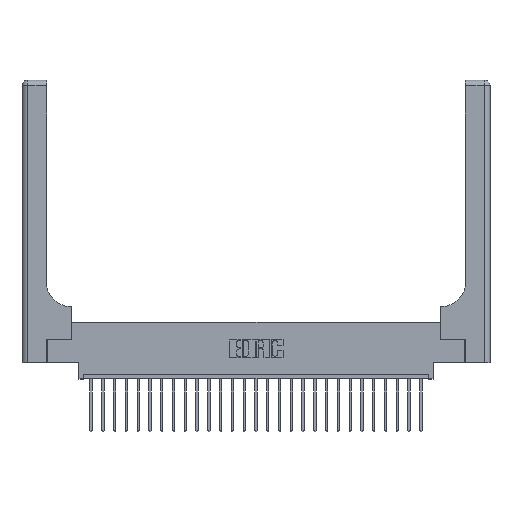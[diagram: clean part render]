
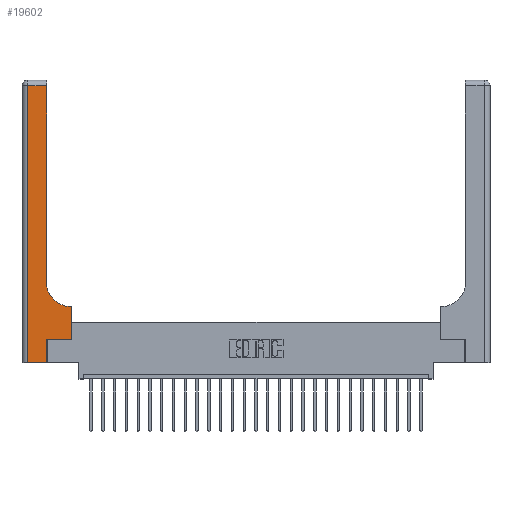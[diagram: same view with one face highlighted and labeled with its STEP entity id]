
A CAD part, top view. The second image highlights one B-rep face of the part: STEP entity #19602.
In plain terms, the highlighted planar face has unit normal (0, 0, 1).
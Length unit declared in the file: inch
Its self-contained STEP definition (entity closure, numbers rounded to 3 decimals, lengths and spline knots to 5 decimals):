
#7 = VERTEX_POINT ( 'NONE', #24614 ) ;
#90 = LINE ( 'NONE', #17116, #2806 ) ;
#502 = VERTEX_POINT ( 'NONE', #16715 ) ;
#616 = PLANE ( 'NONE',  #24711 ) ;
#1683 = ORIENTED_EDGE ( 'NONE', *, *, #7951, .T. ) ;
#2126 = DIRECTION ( 'NONE',  ( 0., 1., 0. ) ) ;
#2358 = LINE ( 'NONE', #4135, #21778 ) ;
#2382 = CARTESIAN_POINT ( 'NONE',  ( 0., 3., 0.37 ) ) ;
#2388 = CARTESIAN_POINT ( 'NONE',  ( 0.528, 0.6, 0.37 ) ) ;
#2448 = CARTESIAN_POINT ( 'NONE',  ( 0.06, 0., 0.37 ) ) ;
#2623 = VECTOR ( 'NONE', #8365, 39.37008 ) ;
#2806 = VECTOR ( 'NONE', #23142, 39.37008 ) ;
#3289 = VECTOR ( 'NONE', #11785, 39.37008 ) ;
#3320 = FACE_OUTER_BOUND ( 'NONE', #7994, .T. ) ;
#3409 = DIRECTION ( 'NONE',  ( -1., 0., 0. ) ) ;
#3862 = VERTEX_POINT ( 'NONE', #4195 ) ;
#4135 = CARTESIAN_POINT ( 'NONE',  ( 0., 0., 0.37 ) ) ;
#4195 = CARTESIAN_POINT ( 'NONE',  ( 0.528, 0.25, 0.37 ) ) ;
#4690 = LINE ( 'NONE', #22848, #9230 ) ;
#5339 = DIRECTION ( 'NONE',  ( 0., 1., 0. ) ) ;
#5441 = EDGE_CURVE ( 'NONE', #12566, #9468, #6853, .T. ) ;
#5526 = ORIENTED_EDGE ( 'NONE', *, *, #9275, .T. ) ;
#6209 = EDGE_CURVE ( 'NONE', #7, #12091, #24894, .T. ) ;
#6340 = DIRECTION ( 'NONE',  ( 0., 0., -1. ) ) ;
#6690 = EDGE_CURVE ( 'NONE', #502, #6794, #16991, .T. ) ;
#6794 = VERTEX_POINT ( 'NONE', #2448 ) ;
#6853 = LINE ( 'NONE', #17221, #7756 ) ;
#7430 = ORIENTED_EDGE ( 'NONE', *, *, #6690, .T. ) ;
#7756 = VECTOR ( 'NONE', #5339, 39.37008 ) ;
#7951 = EDGE_CURVE ( 'NONE', #3862, #21310, #11761, .T. ) ;
#7994 = EDGE_LOOP ( 'NONE', ( #20441, #13271, #7430, #24836, #15666, #5526, #1683, #21961, #8449 ) ) ;
#8229 = CARTESIAN_POINT ( 'NONE',  ( 0.06, 3., 0.37 ) ) ;
#8365 = DIRECTION ( 'NONE',  ( 1., 0., 0. ) ) ;
#8449 = ORIENTED_EDGE ( 'NONE', *, *, #6209, .T. ) ;
#8868 = EDGE_CURVE ( 'NONE', #6794, #12566, #2358, .T. ) ;
#9230 = VECTOR ( 'NONE', #3409, 39.37008 ) ;
#9275 = EDGE_CURVE ( 'NONE', #9468, #3862, #23871, .T. ) ;
#9468 = VERTEX_POINT ( 'NONE', #16492 ) ;
#9527 = CARTESIAN_POINT ( 'NONE',  ( 0.51, 0.85, 0.37 ) ) ;
#11761 = LINE ( 'NONE', #23405, #17508 ) ;
#11785 = DIRECTION ( 'NONE',  ( -1., 0., 0. ) ) ;
#11792 = EDGE_CURVE ( 'NONE', #12091, #20217, #90, .T. ) ;
#12091 = VERTEX_POINT ( 'NONE', #21866 ) ;
#12566 = VERTEX_POINT ( 'NONE', #21459 ) ;
#13271 = ORIENTED_EDGE ( 'NONE', *, *, #19546, .T. ) ;
#13413 = DIRECTION ( 'NONE',  ( 1., 0., 0. ) ) ;
#14569 = VECTOR ( 'NONE', #23489, 39.37008 ) ;
#15497 = DIRECTION ( 'NONE',  ( 0., 0., -1. ) ) ;
#15666 = ORIENTED_EDGE ( 'NONE', *, *, #5441, .T. ) ;
#15782 = EDGE_CURVE ( 'NONE', #21310, #7, #4690, .T. ) ;
#15937 = DIRECTION ( 'NONE',  ( -1., 0., 0. ) ) ;
#16492 = CARTESIAN_POINT ( 'NONE',  ( 0.265, 0.25, 0.37 ) ) ;
#16715 = CARTESIAN_POINT ( 'NONE',  ( 0.06, 2.94, 0.37 ) ) ;
#16991 = LINE ( 'NONE', #8229, #14569 ) ;
#17116 = CARTESIAN_POINT ( 'NONE',  ( 0.26, 3., 0.37 ) ) ;
#17221 = CARTESIAN_POINT ( 'NONE',  ( 0.265, 0., 0.37 ) ) ;
#17508 = VECTOR ( 'NONE', #2126, 39.37008 ) ;
#19519 = CARTESIAN_POINT ( 'NONE',  ( 0., 2.94, 0.37 ) ) ;
#19546 = EDGE_CURVE ( 'NONE', #20217, #502, #23955, .T. ) ;
#19602 = ADVANCED_FACE ( 'NONE', ( #3320 ), #616, .F. ) ;
#19836 = DIRECTION ( 'NONE',  ( 1., 0., 0. ) ) ;
#20217 = VERTEX_POINT ( 'NONE', #23534 ) ;
#20441 = ORIENTED_EDGE ( 'NONE', *, *, #11792, .T. ) ;
#20919 = CARTESIAN_POINT ( 'NONE',  ( 0.265, 0.25, 0.37 ) ) ;
#21310 = VERTEX_POINT ( 'NONE', #2388 ) ;
#21459 = CARTESIAN_POINT ( 'NONE',  ( 0.265, 0., 0.37 ) ) ;
#21778 = VECTOR ( 'NONE', #19836, 39.37008 ) ;
#21866 = CARTESIAN_POINT ( 'NONE',  ( 0.26, 0.85, 0.37 ) ) ;
#21961 = ORIENTED_EDGE ( 'NONE', *, *, #15782, .T. ) ;
#22848 = CARTESIAN_POINT ( 'NONE',  ( 0.26, 0.6, 0.37 ) ) ;
#23142 = DIRECTION ( 'NONE',  ( 0., 1., 0. ) ) ;
#23187 = AXIS2_PLACEMENT_3D ( 'NONE', #9527, #15497, #13413 ) ;
#23405 = CARTESIAN_POINT ( 'NONE',  ( 0.528, 0.25, 0.37 ) ) ;
#23489 = DIRECTION ( 'NONE',  ( 0., -1., 0. ) ) ;
#23534 = CARTESIAN_POINT ( 'NONE',  ( 0.26, 2.94, 0.37 ) ) ;
#23871 = LINE ( 'NONE', #20919, #2623 ) ;
#23955 = LINE ( 'NONE', #19519, #3289 ) ;
#24614 = CARTESIAN_POINT ( 'NONE',  ( 0.51, 0.6, 0.37 ) ) ;
#24711 = AXIS2_PLACEMENT_3D ( 'NONE', #2382, #6340, #15937 ) ;
#24836 = ORIENTED_EDGE ( 'NONE', *, *, #8868, .T. ) ;
#24894 = CIRCLE ( 'NONE', #23187, 0.25 ) ;
